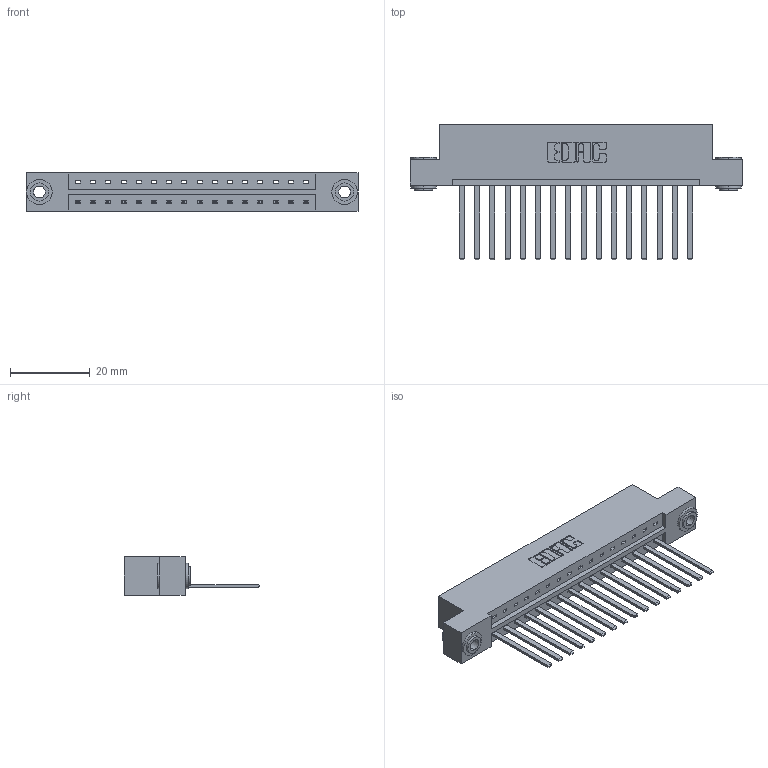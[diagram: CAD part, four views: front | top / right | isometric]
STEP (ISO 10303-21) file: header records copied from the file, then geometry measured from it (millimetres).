
FILE_DESCRIPTION (( 'STEP AP203' ), '1' );
FILE_NAME ('379-016-544-103.STEP', '2020-09-30T16:47:55', ( '' ), ( '' ), 'SwSTEP 2.0', 'SolidWorks 2020', '' );
FILE_SCHEMA (( 'CONFIG_CONTROL_DESIGN' ));
Length unit declared in the file: inch
Products named in the file (4): 345-250-002_345-250-002-102; 379-016-544-103; 379 Part_Flush - .156 Dia - TH; 345-292-001_345-293-144
Assembly tree (19 placements, depth 2):
  379-016-544-103
    379 Part_Flush - .156 Dia - TH
    345-292-001_345-293-144  x16
    345-250-002_345-250-002-102  x2
Bounding box: 83.19 x 33.96 x 9.53 mm (x, y, z)
Volume: 8634.7 mm3; surface area: 9549.7 mm2
Topology: 19 solids, 19 shells, 984 faces, 2915 edges, 1918 vertices
Faces by surface type: plane 688, cylinder 288, cone 8
Entity records: 13610 total; most frequent: CARTESIAN_POINT 2329, ORIENTED_EDGE 2274, DIRECTION 2047, EDGE_CURVE 1137, VECTOR 989, LINE 989, VERTEX_POINT 754, AXIS2_PLACEMENT_3D 529
